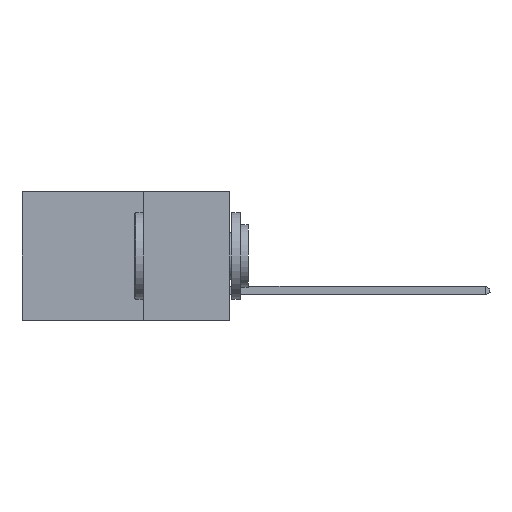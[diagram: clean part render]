
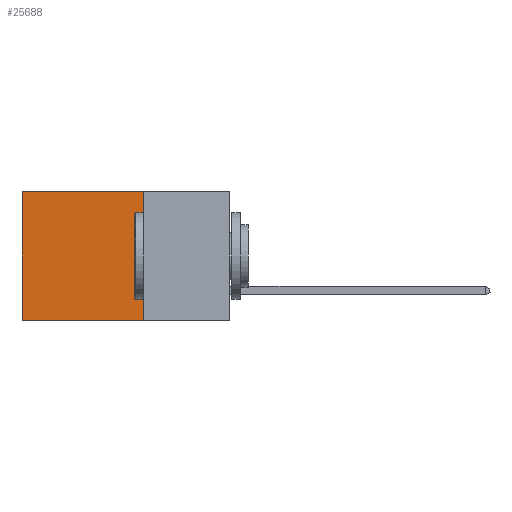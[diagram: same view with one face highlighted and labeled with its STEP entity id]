
A CAD part, left-side view. The second image highlights one B-rep face of the part: STEP entity #25688.
In plain terms, the highlighted planar face has unit normal (-1, 0, 0).
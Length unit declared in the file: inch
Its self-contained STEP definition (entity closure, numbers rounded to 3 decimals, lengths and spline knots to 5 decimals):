
#1667 = DIRECTION ( 'NONE',  ( 0., 1., 0. ) ) ;
#1876 = ORIENTED_EDGE ( 'NONE', *, *, #9489, .F. ) ;
#2082 = VECTOR ( 'NONE', #15695, 39.37008 ) ;
#3933 = CARTESIAN_POINT ( 'NONE',  ( 0.298, 0.25, 0. ) ) ;
#4498 = VECTOR ( 'NONE', #15217, 39.37008 ) ;
#4776 = LINE ( 'NONE', #20213, #27767 ) ;
#5052 = VECTOR ( 'NONE', #14374, 39.37008 ) ;
#5867 = VERTEX_POINT ( 'NONE', #8331 ) ;
#5955 = CARTESIAN_POINT ( 'NONE',  ( 0.298, 0.25, 0. ) ) ;
#6343 = CARTESIAN_POINT ( 'NONE',  ( 0.298, 0.25, 0. ) ) ;
#6369 = DIRECTION ( 'NONE',  ( 0., 0., -1. ) ) ;
#8331 = CARTESIAN_POINT ( 'NONE',  ( 0.298, 0.6, -0.37 ) ) ;
#9257 = ORIENTED_EDGE ( 'NONE', *, *, #13193, .T. ) ;
#9489 = EDGE_CURVE ( 'NONE', #27690, #29845, #20673, .T. ) ;
#9841 = LINE ( 'NONE', #21273, #5052 ) ;
#11649 = AXIS2_PLACEMENT_3D ( 'NONE', #3933, #20187, #6369 ) ;
#11667 = EDGE_CURVE ( 'NONE', #20873, #5867, #16883, .T. ) ;
#13193 = EDGE_CURVE ( 'NONE', #27690, #20873, #4776, .T. ) ;
#13743 = CARTESIAN_POINT ( 'NONE',  ( 0.298, 0.6, 0. ) ) ;
#14374 = DIRECTION ( 'NONE',  ( 0., 1., 0. ) ) ;
#15217 = DIRECTION ( 'NONE',  ( 0., 0., -1. ) ) ;
#15695 = DIRECTION ( 'NONE',  ( 0., 0., -1. ) ) ;
#16883 = LINE ( 'NONE', #22012, #4498 ) ;
#16979 = ORIENTED_EDGE ( 'NONE', *, *, #17137, .F. ) ;
#17137 = EDGE_CURVE ( 'NONE', #29845, #5867, #9841, .T. ) ;
#20187 = DIRECTION ( 'NONE',  ( 1., 0., 0. ) ) ;
#20213 = CARTESIAN_POINT ( 'NONE',  ( 0.298, 0.25, 0. ) ) ;
#20673 = LINE ( 'NONE', #6343, #2082 ) ;
#20873 = VERTEX_POINT ( 'NONE', #13743 ) ;
#21094 = ORIENTED_EDGE ( 'NONE', *, *, #11667, .T. ) ;
#21273 = CARTESIAN_POINT ( 'NONE',  ( 0.298, 0.25, -0.37 ) ) ;
#22012 = CARTESIAN_POINT ( 'NONE',  ( 0.298, 0.6, 0. ) ) ;
#22162 = FACE_OUTER_BOUND ( 'NONE', #23203, .T. ) ;
#22411 = PLANE ( 'NONE',  #11649 ) ;
#23203 = EDGE_LOOP ( 'NONE', ( #21094, #16979, #1876, #9257 ) ) ;
#25688 = ADVANCED_FACE ( 'NONE', ( #22162 ), #22411, .F. ) ;
#26645 = CARTESIAN_POINT ( 'NONE',  ( 0.298, 0.25, -0.37 ) ) ;
#27690 = VERTEX_POINT ( 'NONE', #5955 ) ;
#27767 = VECTOR ( 'NONE', #1667, 39.37008 ) ;
#29845 = VERTEX_POINT ( 'NONE', #26645 ) ;
